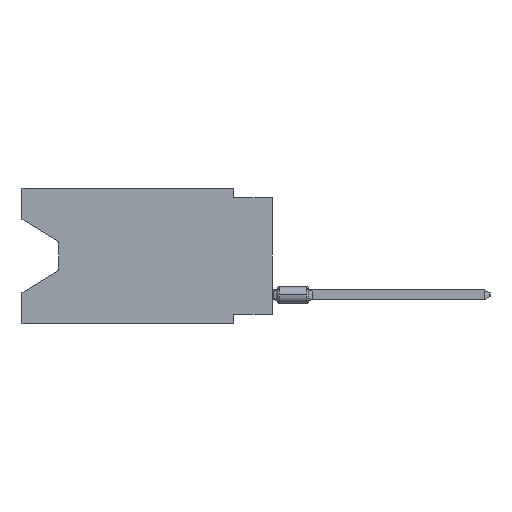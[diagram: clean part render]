
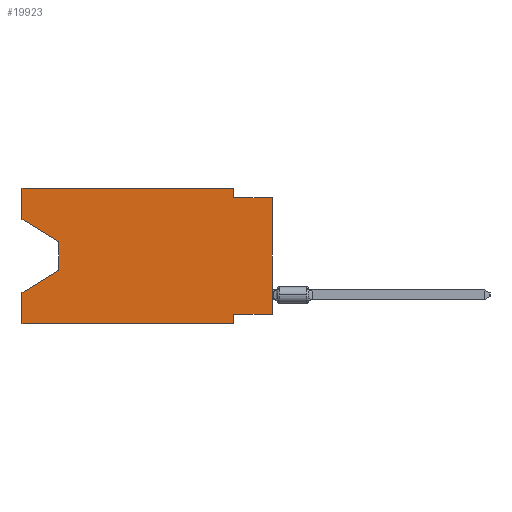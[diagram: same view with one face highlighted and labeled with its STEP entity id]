
A CAD part, left-side view. The second image highlights one B-rep face of the part: STEP entity #19923.
In plain terms, the highlighted planar face has unit normal (-1, 0, 0).
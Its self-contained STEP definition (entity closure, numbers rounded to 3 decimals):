
#149 = EDGE_CURVE ( 'NONE', #18272, #18442, #17932, .T. ) ;
#1409 = CARTESIAN_POINT ( 'NONE',  ( 0., 2.54, -8.255 ) ) ;
#3094 = EDGE_CURVE ( 'NONE', #46281, #64789, #28614, .T. ) ;
#3386 = ORIENTED_EDGE ( 'NONE', *, *, #15524, .F. ) ;
#4226 = CARTESIAN_POINT ( 'NONE',  ( 0., 16.383, 0. ) ) ;
#4961 = CARTESIAN_POINT ( 'NONE',  ( 0., 2.54, -0.635 ) ) ;
#5087 = FACE_OUTER_BOUND ( 'NONE', #55539, .T. ) ;
#6394 = LINE ( 'NONE', #11865, #48819 ) ;
#7104 = LINE ( 'NONE', #64869, #60103 ) ;
#7250 = ORIENTED_EDGE ( 'NONE', *, *, #53906, .F. ) ;
#7265 = CARTESIAN_POINT ( 'NONE',  ( 0., 13.97, -5.385 ) ) ;
#7464 = CARTESIAN_POINT ( 'NONE',  ( 0., 13.97, -3.505 ) ) ;
#7568 = EDGE_CURVE ( 'NONE', #64680, #18272, #6394, .T. ) ;
#7762 = DIRECTION ( 'NONE',  ( 0., 0., -1. ) ) ;
#9202 = CARTESIAN_POINT ( 'NONE',  ( 0., 16.383, 0. ) ) ;
#9513 = ORIENTED_EDGE ( 'NONE', *, *, #49467, .T. ) ;
#10568 = DIRECTION ( 'NONE',  ( 0., 0., -1. ) ) ;
#11865 = CARTESIAN_POINT ( 'NONE',  ( 0., 16.383, -2.038 ) ) ;
#12740 = LINE ( 'NONE', #7265, #49586 ) ;
#12788 = DIRECTION ( 'NONE',  ( 0., 0., -1. ) ) ;
#12945 = CARTESIAN_POINT ( 'NONE',  ( 0., 16.383, 0. ) ) ;
#13292 = LINE ( 'NONE', #12945, #25850 ) ;
#15524 = EDGE_CURVE ( 'NONE', #19573, #46281, #13292, .T. ) ;
#15700 = DIRECTION ( 'NONE',  ( 1., 0., 0. ) ) ;
#17680 = DIRECTION ( 'NONE',  ( 0., -0.855, -0.519 ) ) ;
#17932 = LINE ( 'NONE', #38766, #19819 ) ;
#18272 = VERTEX_POINT ( 'NONE', #7464 ) ;
#18442 = VERTEX_POINT ( 'NONE', #32519 ) ;
#18721 = LINE ( 'NONE', #43979, #27893 ) ;
#18935 = CARTESIAN_POINT ( 'NONE',  ( 0., 16.383, -6.852 ) ) ;
#19573 = VERTEX_POINT ( 'NONE', #4226 ) ;
#19819 = VECTOR ( 'NONE', #12788, 1000. ) ;
#19923 = ADVANCED_FACE ( 'NONE', ( #5087 ), #52275, .F. ) ;
#20648 = EDGE_CURVE ( 'NONE', #42163, #25108, #7104, .T. ) ;
#21078 = CARTESIAN_POINT ( 'NONE',  ( 0., 0., -8.255 ) ) ;
#22007 = DIRECTION ( 'NONE',  ( 0., 0.855, -0.519 ) ) ;
#22103 = VECTOR ( 'NONE', #24253, 1000. ) ;
#22284 = VECTOR ( 'NONE', #7762, 1000. ) ;
#23188 = CARTESIAN_POINT ( 'NONE',  ( 0., 0., -0.635 ) ) ;
#23719 = EDGE_CURVE ( 'NONE', #43241, #60699, #43612, .T. ) ;
#24253 = DIRECTION ( 'NONE',  ( 0., 0., 1. ) ) ;
#25108 = VERTEX_POINT ( 'NONE', #61590 ) ;
#25850 = VECTOR ( 'NONE', #54672, 1000. ) ;
#27227 = DIRECTION ( 'NONE',  ( 0., 0., 1. ) ) ;
#27256 = VECTOR ( 'NONE', #64649, 1000. ) ;
#27893 = VECTOR ( 'NONE', #64844, 1000. ) ;
#28346 = ORIENTED_EDGE ( 'NONE', *, *, #28998, .F. ) ;
#28614 = LINE ( 'NONE', #64843, #22284 ) ;
#28998 = EDGE_CURVE ( 'NONE', #43241, #43581, #35430, .T. ) ;
#30497 = AXIS2_PLACEMENT_3D ( 'NONE', #9202, #15700, #10568 ) ;
#31680 = CARTESIAN_POINT ( 'NONE',  ( 0., 0., 0. ) ) ;
#32099 = VECTOR ( 'NONE', #27227, 1000. ) ;
#32240 = ORIENTED_EDGE ( 'NONE', *, *, #149, .T. ) ;
#32519 = CARTESIAN_POINT ( 'NONE',  ( 0., 13.97, -5.385 ) ) ;
#33399 = VECTOR ( 'NONE', #54904, 1000. ) ;
#34050 = LINE ( 'NONE', #40838, #33399 ) ;
#34441 = DIRECTION ( 'NONE',  ( 0., -1., 0. ) ) ;
#35202 = ORIENTED_EDGE ( 'NONE', *, *, #20648, .T. ) ;
#35217 = ORIENTED_EDGE ( 'NONE', *, *, #59456, .F. ) ;
#35430 = LINE ( 'NONE', #21078, #67381 ) ;
#38766 = CARTESIAN_POINT ( 'NONE',  ( 0., 13.97, -3.505 ) ) ;
#38986 = CARTESIAN_POINT ( 'NONE',  ( 0., 0., -0.635 ) ) ;
#40069 = CARTESIAN_POINT ( 'NONE',  ( 0., 0., -8.255 ) ) ;
#40838 = CARTESIAN_POINT ( 'NONE',  ( 0., 16.383, 0. ) ) ;
#41914 = DIRECTION ( 'NONE',  ( 0., 1., 0. ) ) ;
#42163 = VERTEX_POINT ( 'NONE', #44535 ) ;
#42477 = ORIENTED_EDGE ( 'NONE', *, *, #23719, .T. ) ;
#43241 = VERTEX_POINT ( 'NONE', #40069 ) ;
#43399 = CARTESIAN_POINT ( 'NONE',  ( 0., 2.54, 0. ) ) ;
#43581 = VERTEX_POINT ( 'NONE', #1409 ) ;
#43612 = LINE ( 'NONE', #31680, #32099 ) ;
#43979 = CARTESIAN_POINT ( 'NONE',  ( 0., 2.54, -8.89 ) ) ;
#44535 = CARTESIAN_POINT ( 'NONE',  ( 0., 16.383, -8.89 ) ) ;
#44768 = LINE ( 'NONE', #65626, #22103 ) ;
#45476 = ORIENTED_EDGE ( 'NONE', *, *, #46960, .F. ) ;
#46281 = VERTEX_POINT ( 'NONE', #43399 ) ;
#46960 = EDGE_CURVE ( 'NONE', #43581, #25108, #18721, .T. ) ;
#48819 = VECTOR ( 'NONE', #17680, 1000. ) ;
#49467 = EDGE_CURVE ( 'NONE', #18442, #63787, #12740, .T. ) ;
#49586 = VECTOR ( 'NONE', #22007, 1000. ) ;
#50748 = ORIENTED_EDGE ( 'NONE', *, *, #67055, .F. ) ;
#52230 = ORIENTED_EDGE ( 'NONE', *, *, #3094, .F. ) ;
#52275 = PLANE ( 'NONE',  #30497 ) ;
#53906 = EDGE_CURVE ( 'NONE', #42163, #63787, #34050, .T. ) ;
#54672 = DIRECTION ( 'NONE',  ( 0., -1., 0. ) ) ;
#54904 = DIRECTION ( 'NONE',  ( 0., 0., 1. ) ) ;
#55539 = EDGE_LOOP ( 'NONE', ( #58324, #32240, #9513, #7250, #35202, #45476, #28346, #42477, #35217, #52230, #3386, #50748 ) ) ;
#58324 = ORIENTED_EDGE ( 'NONE', *, *, #7568, .T. ) ;
#59456 = EDGE_CURVE ( 'NONE', #64789, #60699, #60198, .T. ) ;
#60103 = VECTOR ( 'NONE', #34441, 1000. ) ;
#60198 = LINE ( 'NONE', #38986, #27256 ) ;
#60699 = VERTEX_POINT ( 'NONE', #23188 ) ;
#61590 = CARTESIAN_POINT ( 'NONE',  ( 0., 2.54, -8.89 ) ) ;
#62074 = CARTESIAN_POINT ( 'NONE',  ( 0., 16.383, -2.038 ) ) ;
#63787 = VERTEX_POINT ( 'NONE', #18935 ) ;
#64649 = DIRECTION ( 'NONE',  ( 0., -1., 0. ) ) ;
#64680 = VERTEX_POINT ( 'NONE', #62074 ) ;
#64789 = VERTEX_POINT ( 'NONE', #4961 ) ;
#64843 = CARTESIAN_POINT ( 'NONE',  ( 0., 2.54, 0. ) ) ;
#64844 = DIRECTION ( 'NONE',  ( 0., 0., -1. ) ) ;
#64869 = CARTESIAN_POINT ( 'NONE',  ( 0., 16.383, -8.89 ) ) ;
#65626 = CARTESIAN_POINT ( 'NONE',  ( 0., 16.383, 0. ) ) ;
#67055 = EDGE_CURVE ( 'NONE', #64680, #19573, #44768, .T. ) ;
#67381 = VECTOR ( 'NONE', #41914, 1000. ) ;
